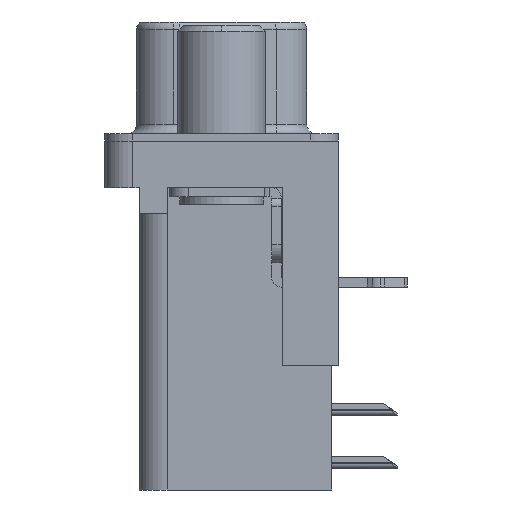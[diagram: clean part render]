
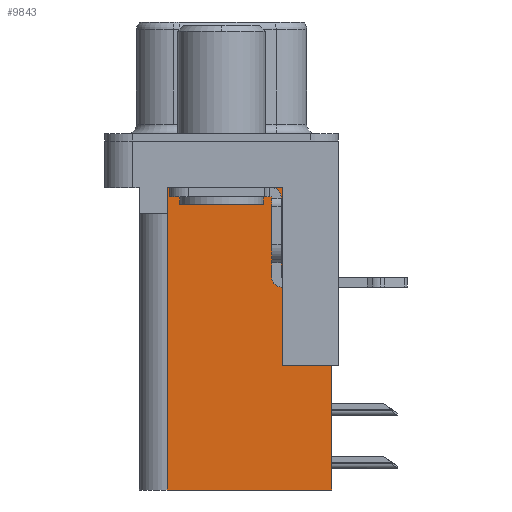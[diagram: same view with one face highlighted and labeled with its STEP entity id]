
A CAD part, left-side view. The second image highlights one B-rep face of the part: STEP entity #9843.
In plain terms, the highlighted planar face has unit normal (-1, 0, 0).
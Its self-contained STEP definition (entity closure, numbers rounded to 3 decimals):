
#26 = FACE_OUTER_BOUND ( 'NONE', #9920, .T. ) ;
#304 = VECTOR ( 'NONE', #23167, 1000. ) ;
#444 = CARTESIAN_POINT ( 'NONE',  ( 3.7, 2.925, -18.76 ) ) ;
#526 = VERTEX_POINT ( 'NONE', #8445 ) ;
#811 = CARTESIAN_POINT ( 'NONE',  ( 3.7, -5.925, -2. ) ) ;
#990 = LINE ( 'NONE', #1814, #304 ) ;
#1059 = VERTEX_POINT ( 'NONE', #7591 ) ;
#1301 = CARTESIAN_POINT ( 'NONE',  ( 3.7, 2.895, -3.9 ) ) ;
#1520 = CARTESIAN_POINT ( 'NONE',  ( 3.7, -3.295, -18.76 ) ) ;
#1669 = VECTOR ( 'NONE', #8987, 1000. ) ;
#1693 = LINE ( 'NONE', #17889, #1669 ) ;
#1814 = CARTESIAN_POINT ( 'NONE',  ( 3.7, 2.895, -3.9 ) ) ;
#2021 = CARTESIAN_POINT ( 'NONE',  ( 3.7, -5.925, -12.05 ) ) ;
#2233 = VECTOR ( 'NONE', #15356, 1000. ) ;
#2542 = CARTESIAN_POINT ( 'NONE',  ( 3.7, 0., -3.9 ) ) ;
#3301 = LINE ( 'NONE', #811, #2233 ) ;
#3583 = VERTEX_POINT ( 'NONE', #6720 ) ;
#4018 = VECTOR ( 'NONE', #13081, 1000. ) ;
#4364 = AXIS2_PLACEMENT_3D ( 'NONE', #1520, #17827, #6995 ) ;
#4547 = LINE ( 'NONE', #11267, #4018 ) ;
#4930 = CARTESIAN_POINT ( 'NONE',  ( 3.7, -5.925, -18.76 ) ) ;
#5431 = EDGE_CURVE ( 'NONE', #1059, #8641, #990, .T. ) ;
#5728 = VECTOR ( 'NONE', #18977, 1000. ) ;
#5792 = LINE ( 'NONE', #2542, #5728 ) ;
#6322 = ORIENTED_EDGE ( 'NONE', *, *, #8631, .T. ) ;
#6594 = CARTESIAN_POINT ( 'NONE',  ( 3.7, -3.295, -18.76 ) ) ;
#6718 = VERTEX_POINT ( 'NONE', #22863 ) ;
#6720 = CARTESIAN_POINT ( 'NONE',  ( 3.7, -3.295, -12.05 ) ) ;
#6995 = DIRECTION ( 'NONE',  ( 0., 1., 0. ) ) ;
#7040 = EDGE_CURVE ( 'NONE', #23406, #18531, #4547, .T. ) ;
#7591 = CARTESIAN_POINT ( 'NONE',  ( 3.7, 2.895, -2.5 ) ) ;
#8110 = EDGE_CURVE ( 'NONE', #21105, #3583, #1693, .T. ) ;
#8445 = CARTESIAN_POINT ( 'NONE',  ( 3.7, 2.925, -3.9 ) ) ;
#8479 = EDGE_CURVE ( 'NONE', #21105, #23406, #3301, .T. ) ;
#8631 = EDGE_CURVE ( 'NONE', #3583, #6718, #19876, .T. ) ;
#8641 = VERTEX_POINT ( 'NONE', #1301 ) ;
#8783 = EDGE_CURVE ( 'NONE', #18531, #526, #15621, .T. ) ;
#8987 = DIRECTION ( 'NONE',  ( 0., 1., 0. ) ) ;
#9843 = ADVANCED_FACE ( 'NONE', ( #26 ), #12544, .F. ) ;
#9920 = EDGE_LOOP ( 'NONE', ( #15037, #17871, #14918, #17316, #19805, #21544, #21363, #6322 ) ) ;
#10435 = DIRECTION ( 'NONE',  ( 0., 0., 1. ) ) ;
#10881 = DIRECTION ( 'NONE',  ( 0., 1., 0. ) ) ;
#11267 = CARTESIAN_POINT ( 'NONE',  ( 3.7, -3.295, -18.76 ) ) ;
#12544 = PLANE ( 'NONE',  #4364 ) ;
#13081 = DIRECTION ( 'NONE',  ( 0., 1., 0. ) ) ;
#14918 = ORIENTED_EDGE ( 'NONE', *, *, #23201, .T. ) ;
#15037 = ORIENTED_EDGE ( 'NONE', *, *, #20446, .T. ) ;
#15356 = DIRECTION ( 'NONE',  ( 0., 0., -1. ) ) ;
#15412 = CARTESIAN_POINT ( 'NONE',  ( 3.7, 2.925, -18.76 ) ) ;
#15621 = LINE ( 'NONE', #15412, #18169 ) ;
#17218 = DIRECTION ( 'NONE',  ( 0., 0., 1. ) ) ;
#17316 = ORIENTED_EDGE ( 'NONE', *, *, #8783, .F. ) ;
#17827 = DIRECTION ( 'NONE',  ( 1., 0., 0. ) ) ;
#17871 = ORIENTED_EDGE ( 'NONE', *, *, #5431, .T. ) ;
#17889 = CARTESIAN_POINT ( 'NONE',  ( 3.7, -6.295, -12.05 ) ) ;
#18169 = VECTOR ( 'NONE', #17218, 1000. ) ;
#18531 = VERTEX_POINT ( 'NONE', #444 ) ;
#18977 = DIRECTION ( 'NONE',  ( 0., 1., 0. ) ) ;
#19015 = VECTOR ( 'NONE', #10435, 1000. ) ;
#19805 = ORIENTED_EDGE ( 'NONE', *, *, #7040, .F. ) ;
#19876 = LINE ( 'NONE', #6594, #19015 ) ;
#20446 = EDGE_CURVE ( 'NONE', #6718, #1059, #21586, .T. ) ;
#21105 = VERTEX_POINT ( 'NONE', #2021 ) ;
#21363 = ORIENTED_EDGE ( 'NONE', *, *, #8110, .T. ) ;
#21544 = ORIENTED_EDGE ( 'NONE', *, *, #8479, .F. ) ;
#21561 = CARTESIAN_POINT ( 'NONE',  ( 3.7, -3.295, -2.5 ) ) ;
#21586 = LINE ( 'NONE', #21561, #21899 ) ;
#21899 = VECTOR ( 'NONE', #10881, 1000. ) ;
#22863 = CARTESIAN_POINT ( 'NONE',  ( 3.7, -3.295, -2.5 ) ) ;
#23167 = DIRECTION ( 'NONE',  ( 0., 0., -1. ) ) ;
#23201 = EDGE_CURVE ( 'NONE', #8641, #526, #5792, .T. ) ;
#23406 = VERTEX_POINT ( 'NONE', #4930 ) ;
